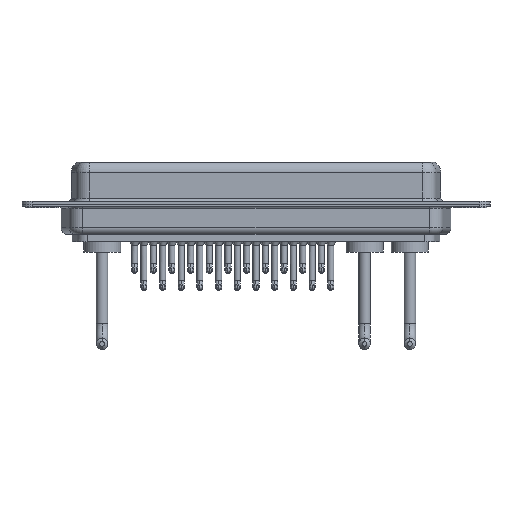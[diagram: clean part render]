
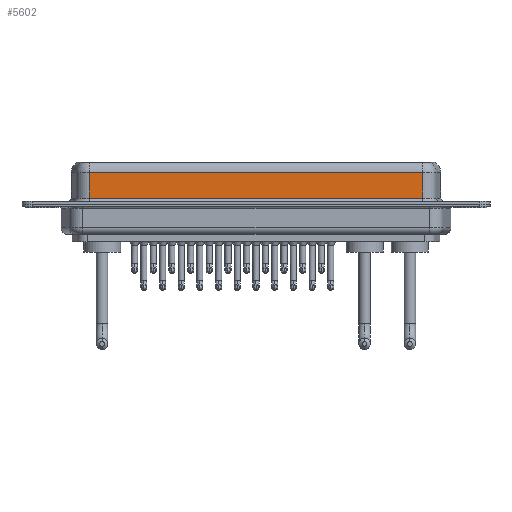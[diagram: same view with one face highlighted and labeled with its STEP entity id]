
A CAD part, front view. The second image highlights one B-rep face of the part: STEP entity #5602.
In plain terms, the highlighted planar face has unit normal (0, -1, 0).
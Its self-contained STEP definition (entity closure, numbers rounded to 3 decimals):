
#264 = EDGE_CURVE ( 'NONE', #19204, #6319, #16379, .T. ) ;
#713 = DIRECTION ( 'NONE',  ( -1., 0., 0. ) ) ;
#1889 = CARTESIAN_POINT ( 'NONE',  ( 56.462, -3.95, 0.9 ) ) ;
#2150 = ORIENTED_EDGE ( 'NONE', *, *, #11568, .T. ) ;
#3094 = VERTEX_POINT ( 'NONE', #19801 ) ;
#4377 = AXIS2_PLACEMENT_3D ( 'NONE', #20915, #17564, #17452 ) ;
#4985 = CARTESIAN_POINT ( 'NONE',  ( 56.462, -3.95, 6.4 ) ) ;
#5015 = CARTESIAN_POINT ( 'NONE',  ( 7.038, -3.95, 0.9 ) ) ;
#5602 = ADVANCED_FACE ( 'NONE', ( #21021 ), #10656, .F. ) ;
#5819 = ORIENTED_EDGE ( 'NONE', *, *, #264, .T. ) ;
#6103 = VECTOR ( 'NONE', #8726, 1000. ) ;
#6319 = VERTEX_POINT ( 'NONE', #1889 ) ;
#7438 = VERTEX_POINT ( 'NONE', #10522 ) ;
#7595 = ORIENTED_EDGE ( 'NONE', *, *, #9352, .F. ) ;
#8726 = DIRECTION ( 'NONE',  ( 0., 0., -1. ) ) ;
#9352 = EDGE_CURVE ( 'NONE', #3094, #6319, #13480, .T. ) ;
#9689 = CARTESIAN_POINT ( 'NONE',  ( 56.462, -3.95, 0.9 ) ) ;
#10017 = DIRECTION ( 'NONE',  ( 1., 0., 0. ) ) ;
#10522 = CARTESIAN_POINT ( 'NONE',  ( 7.038, -3.95, 4.65 ) ) ;
#10656 = PLANE ( 'NONE',  #4377 ) ;
#10825 = CARTESIAN_POINT ( 'NONE',  ( 7.038, -3.95, 6.4 ) ) ;
#11568 = EDGE_CURVE ( 'NONE', #3094, #7438, #18982, .T. ) ;
#12127 = ORIENTED_EDGE ( 'NONE', *, *, #15574, .T. ) ;
#13254 = DIRECTION ( 'NONE',  ( 0., 0., -1. ) ) ;
#13480 = LINE ( 'NONE', #4985, #20146 ) ;
#15364 = VECTOR ( 'NONE', #10017, 1000. ) ;
#15574 = EDGE_CURVE ( 'NONE', #7438, #19204, #20868, .T. ) ;
#15618 = EDGE_LOOP ( 'NONE', ( #7595, #2150, #12127, #5819 ) ) ;
#15977 = CARTESIAN_POINT ( 'NONE',  ( 56.462, -3.95, 4.65 ) ) ;
#16379 = LINE ( 'NONE', #9689, #15364 ) ;
#17452 = DIRECTION ( 'NONE',  ( 0., 0., 1. ) ) ;
#17564 = DIRECTION ( 'NONE',  ( 0., 1., 0. ) ) ;
#18982 = LINE ( 'NONE', #15977, #20916 ) ;
#19204 = VERTEX_POINT ( 'NONE', #5015 ) ;
#19801 = CARTESIAN_POINT ( 'NONE',  ( 56.462, -3.95, 4.65 ) ) ;
#20146 = VECTOR ( 'NONE', #13254, 1000. ) ;
#20868 = LINE ( 'NONE', #10825, #6103 ) ;
#20915 = CARTESIAN_POINT ( 'NONE',  ( 56.462, -3.95, 6.4 ) ) ;
#20916 = VECTOR ( 'NONE', #713, 1000. ) ;
#21021 = FACE_OUTER_BOUND ( 'NONE', #15618, .T. ) ;
